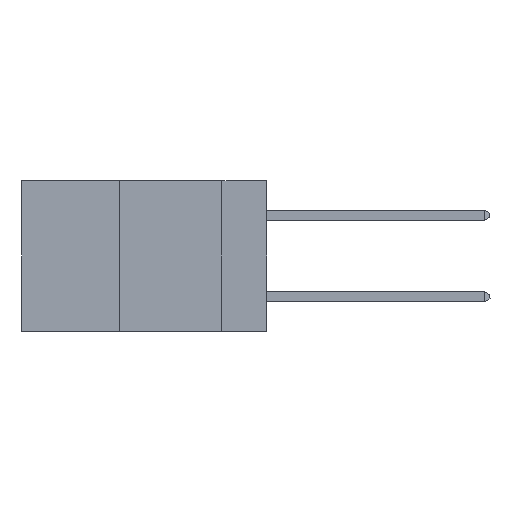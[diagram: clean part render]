
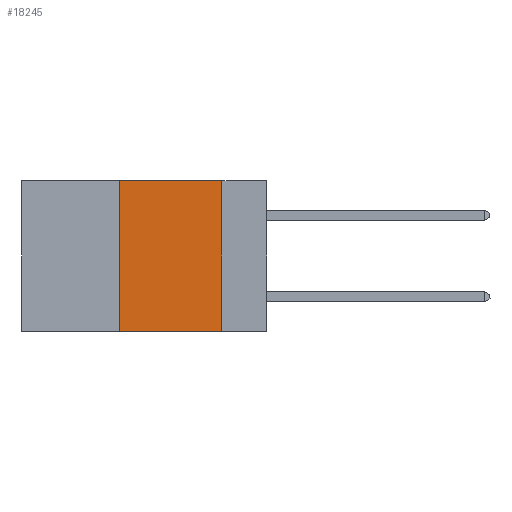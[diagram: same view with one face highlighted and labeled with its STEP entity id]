
A CAD part, left-side view. The second image highlights one B-rep face of the part: STEP entity #18245.
In plain terms, the highlighted planar face has unit normal (-1, 0, 0).
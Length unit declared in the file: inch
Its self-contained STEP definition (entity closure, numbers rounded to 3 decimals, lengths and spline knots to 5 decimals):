
#810 = VECTOR ( 'NONE', #1892, 39.37008 ) ;
#830 = CARTESIAN_POINT ( 'NONE',  ( 0., 0.36, -0.37 ) ) ;
#1882 = DIRECTION ( 'NONE',  ( 1., 0., 0. ) ) ;
#1892 = DIRECTION ( 'NONE',  ( 0., -1., 0. ) ) ;
#2580 = VECTOR ( 'NONE', #14514, 39.37008 ) ;
#2731 = EDGE_CURVE ( 'NONE', #3511, #3813, #8954, .T. ) ;
#3511 = VERTEX_POINT ( 'NONE', #7963 ) ;
#3813 = VERTEX_POINT ( 'NONE', #18561 ) ;
#3844 = CARTESIAN_POINT ( 'NONE',  ( 0., 0.11, 0. ) ) ;
#4221 = EDGE_LOOP ( 'NONE', ( #11860, #4753, #16652, #13724 ) ) ;
#4469 = CARTESIAN_POINT ( 'NONE',  ( 0., 0.36, 0. ) ) ;
#4753 = ORIENTED_EDGE ( 'NONE', *, *, #2731, .F. ) ;
#4921 = AXIS2_PLACEMENT_3D ( 'NONE', #10505, #1882, #11929 ) ;
#5436 = CARTESIAN_POINT ( 'NONE',  ( 0., 0.6, -0.37 ) ) ;
#5540 = VECTOR ( 'NONE', #12400, 39.37008 ) ;
#6240 = PLANE ( 'NONE',  #4921 ) ;
#6627 = VERTEX_POINT ( 'NONE', #830 ) ;
#7549 = VERTEX_POINT ( 'NONE', #17659 ) ;
#7963 = CARTESIAN_POINT ( 'NONE',  ( 0., 0.36, 0. ) ) ;
#8954 = LINE ( 'NONE', #13421, #810 ) ;
#10505 = CARTESIAN_POINT ( 'NONE',  ( 0., 0.6, 0. ) ) ;
#10627 = EDGE_CURVE ( 'NONE', #6627, #7549, #17467, .T. ) ;
#11860 = ORIENTED_EDGE ( 'NONE', *, *, #16439, .F. ) ;
#11929 = DIRECTION ( 'NONE',  ( 0., 0., -1. ) ) ;
#12400 = DIRECTION ( 'NONE',  ( 0., 0., -1. ) ) ;
#13421 = CARTESIAN_POINT ( 'NONE',  ( 0., 0.6, 0. ) ) ;
#13623 = VECTOR ( 'NONE', #16902, 39.37008 ) ;
#13724 = ORIENTED_EDGE ( 'NONE', *, *, #10627, .T. ) ;
#14514 = DIRECTION ( 'NONE',  ( 0., 0., 1. ) ) ;
#15503 = EDGE_CURVE ( 'NONE', #6627, #3511, #17454, .T. ) ;
#16439 = EDGE_CURVE ( 'NONE', #3813, #7549, #16500, .T. ) ;
#16500 = LINE ( 'NONE', #3844, #5540 ) ;
#16652 = ORIENTED_EDGE ( 'NONE', *, *, #15503, .F. ) ;
#16902 = DIRECTION ( 'NONE',  ( 0., -1., 0. ) ) ;
#17454 = LINE ( 'NONE', #4469, #2580 ) ;
#17467 = LINE ( 'NONE', #5436, #13623 ) ;
#17659 = CARTESIAN_POINT ( 'NONE',  ( 0., 0.11, -0.37 ) ) ;
#17990 = FACE_OUTER_BOUND ( 'NONE', #4221, .T. ) ;
#18245 = ADVANCED_FACE ( 'NONE', ( #17990 ), #6240, .F. ) ;
#18561 = CARTESIAN_POINT ( 'NONE',  ( 0., 0.11, 0. ) ) ;
